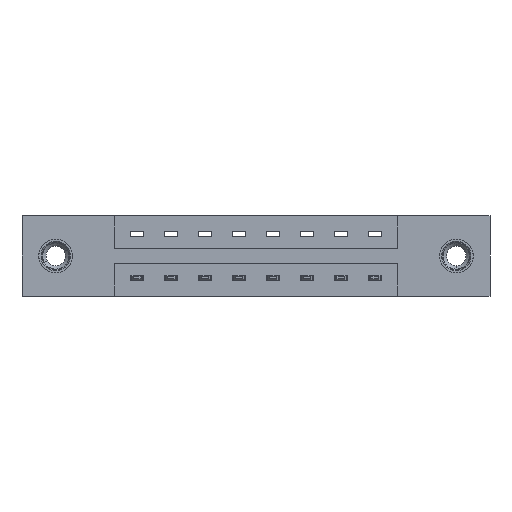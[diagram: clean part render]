
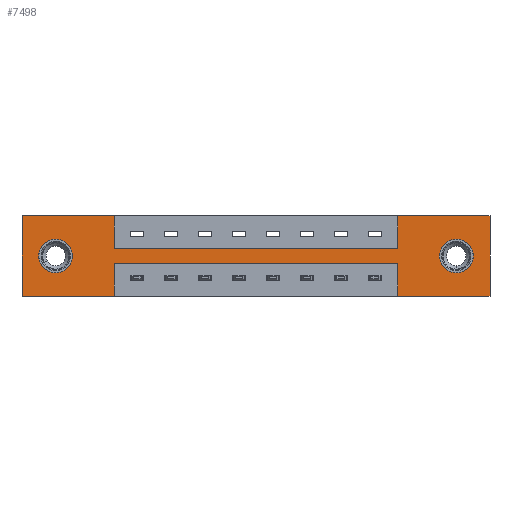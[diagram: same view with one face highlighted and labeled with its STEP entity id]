
A CAD part, front view. The second image highlights one B-rep face of the part: STEP entity #7498.
In plain terms, the highlighted planar face has unit normal (0, -1, 0).
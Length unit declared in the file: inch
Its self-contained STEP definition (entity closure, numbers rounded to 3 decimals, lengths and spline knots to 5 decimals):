
#15 = AXIS2_PLACEMENT_3D ( 'NONE', #4078, #9930, #4964 ) ;
#33 = DIRECTION ( 'NONE',  ( 0., 0., -1. ) ) ;
#282 = DIRECTION ( 'NONE',  ( 1., 0., 0. ) ) ;
#416 = EDGE_CURVE ( 'NONE', #2560, #2083, #10636, .T. ) ;
#484 = EDGE_CURVE ( 'NONE', #2083, #1725, #7485, .T. ) ;
#684 = CARTESIAN_POINT ( 'NONE',  ( 2.154, 0., 0. ) ) ;
#704 = CARTESIAN_POINT ( 'NONE',  ( 0.425, 0., -0.37 ) ) ;
#899 = DIRECTION ( 'NONE',  ( -1., 0., 0. ) ) ;
#945 = VERTEX_POINT ( 'NONE', #9654 ) ;
#951 = LINE ( 'NONE', #11016, #7912 ) ;
#1058 = CARTESIAN_POINT ( 'NONE',  ( 1.729, 0., -0.15 ) ) ;
#1097 = LINE ( 'NONE', #9738, #3404 ) ;
#1187 = CARTESIAN_POINT ( 'NONE',  ( 1.729, 0., -0.37 ) ) ;
#1323 = CARTESIAN_POINT ( 'NONE',  ( 0., 0., 0. ) ) ;
#1365 = CARTESIAN_POINT ( 'NONE',  ( 1.999, 0., -0.185 ) ) ;
#1654 = LINE ( 'NONE', #7581, #6313 ) ;
#1663 = ORIENTED_EDGE ( 'NONE', *, *, #9796, .T. ) ;
#1687 = ORIENTED_EDGE ( 'NONE', *, *, #7292, .T. ) ;
#1700 = ORIENTED_EDGE ( 'NONE', *, *, #3637, .T. ) ;
#1725 = VERTEX_POINT ( 'NONE', #3419 ) ;
#1794 = ORIENTED_EDGE ( 'NONE', *, *, #10272, .T. ) ;
#1841 = ORIENTED_EDGE ( 'NONE', *, *, #3876, .F. ) ;
#1880 = CIRCLE ( 'NONE', #2041, 0.078 ) ;
#1883 = ORIENTED_EDGE ( 'NONE', *, *, #484, .F. ) ;
#1898 = ORIENTED_EDGE ( 'NONE', *, *, #416, .F. ) ;
#1909 = EDGE_LOOP ( 'NONE', ( #1700, #1794 ) ) ;
#1945 = ORIENTED_EDGE ( 'NONE', *, *, #2127, .F. ) ;
#1962 = DIRECTION ( 'NONE',  ( 0., 0., 1. ) ) ;
#2000 = ORIENTED_EDGE ( 'NONE', *, *, #9178, .F. ) ;
#2021 = VERTEX_POINT ( 'NONE', #10179 ) ;
#2041 = AXIS2_PLACEMENT_3D ( 'NONE', #1365, #7696, #2328 ) ;
#2043 = ORIENTED_EDGE ( 'NONE', *, *, #2900, .F. ) ;
#2083 = VERTEX_POINT ( 'NONE', #2158 ) ;
#2093 = ORIENTED_EDGE ( 'NONE', *, *, #7385, .F. ) ;
#2095 = ORIENTED_EDGE ( 'NONE', *, *, #6780, .F. ) ;
#2127 = EDGE_CURVE ( 'NONE', #7489, #2560, #1654, .T. ) ;
#2131 = ORIENTED_EDGE ( 'NONE', *, *, #10500, .F. ) ;
#2158 = CARTESIAN_POINT ( 'NONE',  ( 1.729, 0., -0.22 ) ) ;
#2191 = ORIENTED_EDGE ( 'NONE', *, *, #8583, .F. ) ;
#2267 = ORIENTED_EDGE ( 'NONE', *, *, #10762, .F. ) ;
#2290 = ORIENTED_EDGE ( 'NONE', *, *, #8528, .F. ) ;
#2328 = DIRECTION ( 'NONE',  ( 0., 0., -1. ) ) ;
#2394 = EDGE_LOOP ( 'NONE', ( #1663, #1687 ) ) ;
#2438 = AXIS2_PLACEMENT_3D ( 'NONE', #9610, #5484, #11196 ) ;
#2539 = VERTEX_POINT ( 'NONE', #7026 ) ;
#2560 = VERTEX_POINT ( 'NONE', #8764 ) ;
#2677 = VERTEX_POINT ( 'NONE', #7851 ) ;
#2685 = CARTESIAN_POINT ( 'NONE',  ( 1.999, 0., -0.263 ) ) ;
#2817 = DIRECTION ( 'NONE',  ( 0., 0., 1. ) ) ;
#2900 = EDGE_CURVE ( 'NONE', #2021, #10067, #10953, .T. ) ;
#3073 = CARTESIAN_POINT ( 'NONE',  ( 1.999, 0., -0.107 ) ) ;
#3090 = VERTEX_POINT ( 'NONE', #2685 ) ;
#3136 = VECTOR ( 'NONE', #10286, 39.37008 ) ;
#3163 = DIRECTION ( 'NONE',  ( -1., 0., 0. ) ) ;
#3404 = VECTOR ( 'NONE', #899, 39.37008 ) ;
#3419 = CARTESIAN_POINT ( 'NONE',  ( 0.425, 0., -0.22 ) ) ;
#3621 = VERTEX_POINT ( 'NONE', #1058 ) ;
#3637 = EDGE_CURVE ( 'NONE', #2539, #7047, #10819, .T. ) ;
#3645 = AXIS2_PLACEMENT_3D ( 'NONE', #9556, #10266, #6225 ) ;
#3654 = LINE ( 'NONE', #10992, #10373 ) ;
#3864 = CARTESIAN_POINT ( 'NONE',  ( 0.425, 0., -0.37 ) ) ;
#3876 = EDGE_CURVE ( 'NONE', #1725, #6508, #4337, .T. ) ;
#3985 = CARTESIAN_POINT ( 'NONE',  ( 2.154, 0., 0. ) ) ;
#4078 = CARTESIAN_POINT ( 'NONE',  ( 0.155, 0., -0.185 ) ) ;
#4189 = FACE_BOUND ( 'NONE', #1909, .T. ) ;
#4190 = DIRECTION ( 'NONE',  ( -1., 0., 0. ) ) ;
#4337 = LINE ( 'NONE', #704, #6407 ) ;
#4468 = CARTESIAN_POINT ( 'NONE',  ( 0.425, 0., -0.15 ) ) ;
#4475 = FACE_BOUND ( 'NONE', #2394, .T. ) ;
#4880 = DIRECTION ( 'NONE',  ( 0., 0., -1. ) ) ;
#4964 = DIRECTION ( 'NONE',  ( 0., 0., 1. ) ) ;
#5012 = DIRECTION ( 'NONE',  ( 0., 1., 0. ) ) ;
#5072 = VECTOR ( 'NONE', #1962, 39.37008 ) ;
#5121 = CARTESIAN_POINT ( 'NONE',  ( 0., 0., 0. ) ) ;
#5208 = VECTOR ( 'NONE', #4190, 39.37008 ) ;
#5253 = DIRECTION ( 'NONE',  ( 0., 0., -1. ) ) ;
#5484 = DIRECTION ( 'NONE',  ( 0., -1., 0. ) ) ;
#5658 = CARTESIAN_POINT ( 'NONE',  ( 0.425, 0., -0.22 ) ) ;
#5730 = CARTESIAN_POINT ( 'NONE',  ( 0.155, 0., -0.263 ) ) ;
#5974 = VERTEX_POINT ( 'NONE', #3073 ) ;
#6132 = EDGE_LOOP ( 'NONE', ( #1841, #1883, #1898, #1945, #2000, #2043, #2093, #2095, #2131, #2191, #2267, #2290 ) ) ;
#6225 = DIRECTION ( 'NONE',  ( 0., 0., 1. ) ) ;
#6313 = VECTOR ( 'NONE', #3163, 39.37008 ) ;
#6407 = VECTOR ( 'NONE', #33, 39.37008 ) ;
#6508 = VERTEX_POINT ( 'NONE', #3864 ) ;
#6535 = FACE_OUTER_BOUND ( 'NONE', #6132, .T. ) ;
#6587 = CARTESIAN_POINT ( 'NONE',  ( 0., 0., 0. ) ) ;
#6696 = VECTOR ( 'NONE', #282, 39.37008 ) ;
#6780 = EDGE_CURVE ( 'NONE', #10166, #3621, #10196, .T. ) ;
#7026 = CARTESIAN_POINT ( 'NONE',  ( 0.155, 0., -0.107 ) ) ;
#7047 = VERTEX_POINT ( 'NONE', #5730 ) ;
#7170 = CARTESIAN_POINT ( 'NONE',  ( 2.154, 0., -0.37 ) ) ;
#7271 = VECTOR ( 'NONE', #9805, 39.37008 ) ;
#7292 = EDGE_CURVE ( 'NONE', #3090, #5974, #1880, .T. ) ;
#7383 = LINE ( 'NONE', #3985, #11140 ) ;
#7385 = EDGE_CURVE ( 'NONE', #3621, #2021, #951, .T. ) ;
#7394 = CARTESIAN_POINT ( 'NONE',  ( 0., 0., 0. ) ) ;
#7485 = LINE ( 'NONE', #5658, #5208 ) ;
#7489 = VERTEX_POINT ( 'NONE', #7170 ) ;
#7498 = ADVANCED_FACE ( 'NONE', ( #4475, #4189, #6535 ), #10409, .T. ) ;
#7581 = CARTESIAN_POINT ( 'NONE',  ( 0., 0., -0.37 ) ) ;
#7696 = DIRECTION ( 'NONE',  ( 0., 1., 0. ) ) ;
#7851 = CARTESIAN_POINT ( 'NONE',  ( 0., 0., -0.37 ) ) ;
#7912 = VECTOR ( 'NONE', #8610, 39.37008 ) ;
#8367 = CIRCLE ( 'NONE', #15, 0.078 ) ;
#8528 = EDGE_CURVE ( 'NONE', #6508, #2677, #1097, .T. ) ;
#8582 = AXIS2_PLACEMENT_3D ( 'NONE', #9979, #5012, #10770 ) ;
#8583 = EDGE_CURVE ( 'NONE', #9876, #945, #9673, .T. ) ;
#8610 = DIRECTION ( 'NONE',  ( 0., 0., 1. ) ) ;
#8764 = CARTESIAN_POINT ( 'NONE',  ( 1.729, 0., -0.37 ) ) ;
#8869 = CARTESIAN_POINT ( 'NONE',  ( 0.425, 0., -0.15 ) ) ;
#8901 = CIRCLE ( 'NONE', #8582, 0.078 ) ;
#9178 = EDGE_CURVE ( 'NONE', #10067, #7489, #7383, .T. ) ;
#9556 = CARTESIAN_POINT ( 'NONE',  ( 0.155, 0., -0.185 ) ) ;
#9610 = CARTESIAN_POINT ( 'NONE',  ( 0., 0., -0.37 ) ) ;
#9654 = CARTESIAN_POINT ( 'NONE',  ( 0.425, 0., 0. ) ) ;
#9673 = LINE ( 'NONE', #6587, #7271 ) ;
#9738 = CARTESIAN_POINT ( 'NONE',  ( 0., 0., -0.37 ) ) ;
#9796 = EDGE_CURVE ( 'NONE', #5974, #3090, #8901, .T. ) ;
#9805 = DIRECTION ( 'NONE',  ( 1., 0., 0. ) ) ;
#9876 = VERTEX_POINT ( 'NONE', #5121 ) ;
#9930 = DIRECTION ( 'NONE',  ( 0., 1., 0. ) ) ;
#9979 = CARTESIAN_POINT ( 'NONE',  ( 1.999, 0., -0.185 ) ) ;
#10067 = VERTEX_POINT ( 'NONE', #684 ) ;
#10166 = VERTEX_POINT ( 'NONE', #8869 ) ;
#10179 = CARTESIAN_POINT ( 'NONE',  ( 1.729, 0., 0. ) ) ;
#10196 = LINE ( 'NONE', #4468, #3136 ) ;
#10266 = DIRECTION ( 'NONE',  ( 0., 1., 0. ) ) ;
#10272 = EDGE_CURVE ( 'NONE', #7047, #2539, #8367, .T. ) ;
#10286 = DIRECTION ( 'NONE',  ( 1., 0., 0. ) ) ;
#10373 = VECTOR ( 'NONE', #5253, 39.37008 ) ;
#10387 = VECTOR ( 'NONE', #2817, 39.37008 ) ;
#10409 = PLANE ( 'NONE',  #2438 ) ;
#10500 = EDGE_CURVE ( 'NONE', #945, #10166, #3654, .T. ) ;
#10636 = LINE ( 'NONE', #1187, #10387 ) ;
#10762 = EDGE_CURVE ( 'NONE', #2677, #9876, #11367, .T. ) ;
#10770 = DIRECTION ( 'NONE',  ( 0., 0., -1. ) ) ;
#10819 = CIRCLE ( 'NONE', #3645, 0.078 ) ;
#10953 = LINE ( 'NONE', #1323, #6696 ) ;
#10992 = CARTESIAN_POINT ( 'NONE',  ( 0.425, 0., 0. ) ) ;
#11016 = CARTESIAN_POINT ( 'NONE',  ( 1.729, 0., 0. ) ) ;
#11140 = VECTOR ( 'NONE', #4880, 39.37008 ) ;
#11196 = DIRECTION ( 'NONE',  ( 0., 0., -1. ) ) ;
#11367 = LINE ( 'NONE', #7394, #5072 ) ;
